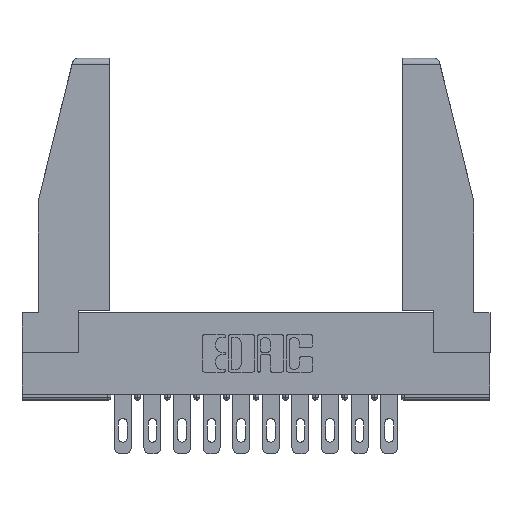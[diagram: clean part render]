
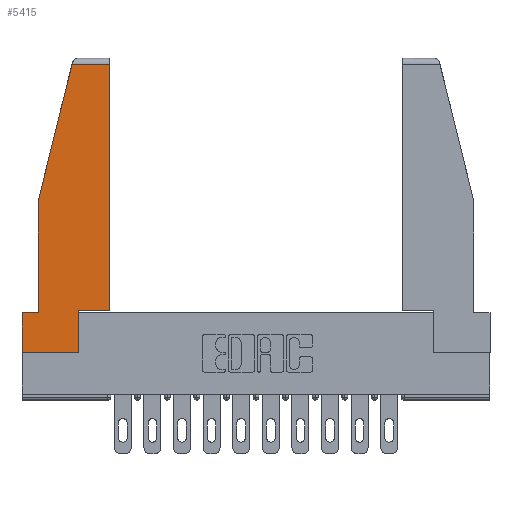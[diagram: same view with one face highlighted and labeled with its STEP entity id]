
A CAD part, top view. The second image highlights one B-rep face of the part: STEP entity #5415.
In plain terms, the highlighted planar face has unit normal (0, 0, 1).
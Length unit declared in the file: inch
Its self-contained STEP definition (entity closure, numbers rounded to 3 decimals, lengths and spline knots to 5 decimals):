
#317 = DIRECTION ( 'NONE',  ( 0., -1., 0. ) ) ;
#363 = LINE ( 'NONE', #8363, #9929 ) ;
#551 = EDGE_CURVE ( 'NONE', #3654, #7751, #8630, .T. ) ;
#901 = LINE ( 'NONE', #4685, #14215 ) ;
#1061 = PLANE ( 'NONE',  #10324 ) ;
#1439 = DIRECTION ( 'NONE',  ( 0., 1., 0. ) ) ;
#1596 = VECTOR ( 'NONE', #317, 39.37008 ) ;
#1772 = DIRECTION ( 'NONE',  ( -0.239, -0.971, 0. ) ) ;
#2104 = VERTEX_POINT ( 'NONE', #2484 ) ;
#2109 = CARTESIAN_POINT ( 'NONE',  ( 0.086, 0.21, 0. ) ) ;
#2162 = ORIENTED_EDGE ( 'NONE', *, *, #10536, .T. ) ;
#2375 = CARTESIAN_POINT ( 'NONE',  ( 0.086, 0.8, 0. ) ) ;
#2484 = CARTESIAN_POINT ( 'NONE',  ( 0.297, 0., 0. ) ) ;
#2814 = LINE ( 'NONE', #12439, #5703 ) ;
#3118 = CARTESIAN_POINT ( 'NONE',  ( 0.461, 0.223, 0. ) ) ;
#3206 = VECTOR ( 'NONE', #10481, 39.37008 ) ;
#3234 = EDGE_CURVE ( 'NONE', #10323, #13226, #901, .T. ) ;
#3423 = CARTESIAN_POINT ( 'NONE',  ( 0.297, 0.223, 0. ) ) ;
#3654 = VERTEX_POINT ( 'NONE', #15636 ) ;
#4016 = EDGE_LOOP ( 'NONE', ( #16435, #6639, #16898, #2162, #8399, #8663, #5340, #7909, #16284 ) ) ;
#4150 = VERTEX_POINT ( 'NONE', #9934 ) ;
#4235 = EDGE_CURVE ( 'NONE', #13226, #4150, #7255, .T. ) ;
#4685 = CARTESIAN_POINT ( 'NONE',  ( 0.297, 0.223, 0. ) ) ;
#5093 = CARTESIAN_POINT ( 'NONE',  ( 0.086, 0.8, 0. ) ) ;
#5173 = VECTOR ( 'NONE', #12438, 39.37008 ) ;
#5340 = ORIENTED_EDGE ( 'NONE', *, *, #8489, .T. ) ;
#5415 = ADVANCED_FACE ( 'NONE', ( #8879 ), #1061, .T. ) ;
#5566 = EDGE_CURVE ( 'NONE', #2104, #10323, #13688, .T. ) ;
#5703 = VECTOR ( 'NONE', #8459, 39.37008 ) ;
#6639 = ORIENTED_EDGE ( 'NONE', *, *, #16775, .T. ) ;
#7255 = LINE ( 'NONE', #3118, #5173 ) ;
#7751 = VERTEX_POINT ( 'NONE', #9031 ) ;
#7909 = ORIENTED_EDGE ( 'NONE', *, *, #5566, .T. ) ;
#8363 = CARTESIAN_POINT ( 'NONE',  ( 0., 1.52, 0. ) ) ;
#8399 = ORIENTED_EDGE ( 'NONE', *, *, #15499, .T. ) ;
#8459 = DIRECTION ( 'NONE',  ( -1., 0., 0. ) ) ;
#8489 = EDGE_CURVE ( 'NONE', #7751, #2104, #8765, .T. ) ;
#8575 = DIRECTION ( 'NONE',  ( 0., 0., 1. ) ) ;
#8630 = LINE ( 'NONE', #14903, #1596 ) ;
#8663 = ORIENTED_EDGE ( 'NONE', *, *, #551, .T. ) ;
#8765 = LINE ( 'NONE', #10646, #13577 ) ;
#8879 = FACE_OUTER_BOUND ( 'NONE', #4016, .T. ) ;
#9031 = CARTESIAN_POINT ( 'NONE',  ( 0., 0., 0. ) ) ;
#9647 = LINE ( 'NONE', #16404, #10924 ) ;
#9839 = DIRECTION ( 'NONE',  ( -1., 0., 0. ) ) ;
#9869 = EDGE_CURVE ( 'NONE', #12805, #13034, #9647, .T. ) ;
#9929 = VECTOR ( 'NONE', #9839, 39.37008 ) ;
#9934 = CARTESIAN_POINT ( 'NONE',  ( 0.461, 1.52, 0. ) ) ;
#9940 = DIRECTION ( 'NONE',  ( 1., 0., 0. ) ) ;
#10323 = VERTEX_POINT ( 'NONE', #3423 ) ;
#10324 = AXIS2_PLACEMENT_3D ( 'NONE', #13954, #8575, #9940 ) ;
#10481 = DIRECTION ( 'NONE',  ( 0., -1., 0. ) ) ;
#10536 = EDGE_CURVE ( 'NONE', #13034, #14182, #11142, .T. ) ;
#10646 = CARTESIAN_POINT ( 'NONE',  ( 0., 0., 0. ) ) ;
#10711 = DIRECTION ( 'NONE',  ( 1., 0., 0. ) ) ;
#10924 = VECTOR ( 'NONE', #1772, 39.37008 ) ;
#11142 = LINE ( 'NONE', #5093, #3206 ) ;
#11711 = CARTESIAN_POINT ( 'NONE',  ( 0.2636, 1.52, 0. ) ) ;
#12438 = DIRECTION ( 'NONE',  ( 0., 1., 0. ) ) ;
#12439 = CARTESIAN_POINT ( 'NONE',  ( 0., 0.21, 0. ) ) ;
#12445 = VECTOR ( 'NONE', #1439, 39.37008 ) ;
#12514 = DIRECTION ( 'NONE',  ( 1., 0., 0. ) ) ;
#12805 = VERTEX_POINT ( 'NONE', #11711 ) ;
#13034 = VERTEX_POINT ( 'NONE', #2375 ) ;
#13226 = VERTEX_POINT ( 'NONE', #14755 ) ;
#13577 = VECTOR ( 'NONE', #10711, 39.37008 ) ;
#13688 = LINE ( 'NONE', #14682, #12445 ) ;
#13954 = CARTESIAN_POINT ( 'NONE',  ( 0., 0., 0. ) ) ;
#14182 = VERTEX_POINT ( 'NONE', #2109 ) ;
#14215 = VECTOR ( 'NONE', #12514, 39.37008 ) ;
#14682 = CARTESIAN_POINT ( 'NONE',  ( 0.297, 0., 0. ) ) ;
#14755 = CARTESIAN_POINT ( 'NONE',  ( 0.461, 0.223, 0. ) ) ;
#14903 = CARTESIAN_POINT ( 'NONE',  ( 0., 0.21, 0. ) ) ;
#15499 = EDGE_CURVE ( 'NONE', #14182, #3654, #2814, .T. ) ;
#15636 = CARTESIAN_POINT ( 'NONE',  ( 0., 0.21, 0. ) ) ;
#16284 = ORIENTED_EDGE ( 'NONE', *, *, #3234, .T. ) ;
#16404 = CARTESIAN_POINT ( 'NONE',  ( 0.271, 1.55, 0. ) ) ;
#16435 = ORIENTED_EDGE ( 'NONE', *, *, #4235, .T. ) ;
#16775 = EDGE_CURVE ( 'NONE', #4150, #12805, #363, .T. ) ;
#16898 = ORIENTED_EDGE ( 'NONE', *, *, #9869, .T. ) ;
